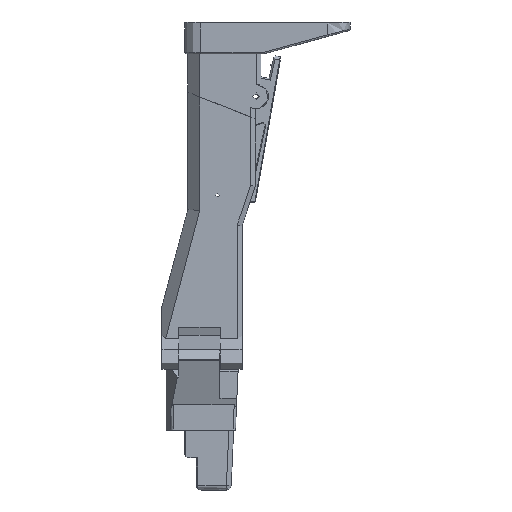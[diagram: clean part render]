
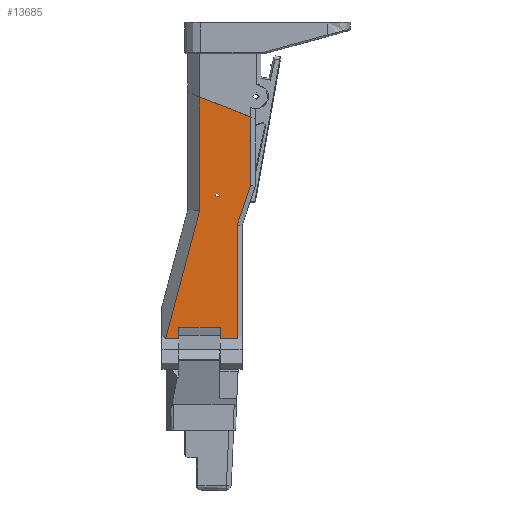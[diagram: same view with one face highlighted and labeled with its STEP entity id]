
A CAD part, left-side view. The second image highlights one B-rep face of the part: STEP entity #13685.
In plain terms, the highlighted planar face has unit normal (-1, 0, 0).
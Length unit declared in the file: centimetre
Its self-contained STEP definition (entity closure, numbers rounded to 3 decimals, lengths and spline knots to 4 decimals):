
#276=FACE_BOUND($,#2141,.T.);
#776=CIRCLE($,#14770,0.11);
#1345=FACE_OUTER_BOUND($,#2140,.T.);
#2140=EDGE_LOOP($,(#10818,#10819,#10820,#10821,#10822,#10823,#10824,#10825,
#10826,#10827,#10828));
#2141=EDGE_LOOP($,(#10829));
#3282=LINE($,#21640,#4736);
#3329=LINE($,#21742,#4783);
#3330=LINE($,#21744,#4784);
#3331=LINE($,#21746,#4785);
#3332=LINE($,#21748,#4786);
#3333=LINE($,#21750,#4787);
#3334=LINE($,#21752,#4788);
#3335=LINE($,#21754,#4789);
#3336=LINE($,#21756,#4790);
#3337=LINE($,#21758,#4791);
#3338=LINE($,#21759,#4792);
#4736=VECTOR($,#17386,3.427);
#4783=VECTOR($,#17457,7.1665);
#4784=VECTOR($,#17458,8.3408);
#4785=VECTOR($,#17459,0.8238);
#4786=VECTOR($,#17460,0.7375);
#4787=VECTOR($,#17461,2.61);
#4788=VECTOR($,#17462,0.7375);
#4789=VECTOR($,#17463,1.075);
#4790=VECTOR($,#17464,7.1624);
#4791=VECTOR($,#17465,2.631);
#4792=VECTOR($,#17466,4.2997);
#6103=VERTEX_POINT($,#21637);
#6104=VERTEX_POINT($,#21639);
#6147=VERTEX_POINT($,#21741);
#6148=VERTEX_POINT($,#21743);
#6149=VERTEX_POINT($,#21745);
#6150=VERTEX_POINT($,#21747);
#6151=VERTEX_POINT($,#21749);
#6152=VERTEX_POINT($,#21751);
#6153=VERTEX_POINT($,#21753);
#6154=VERTEX_POINT($,#21755);
#6155=VERTEX_POINT($,#21757);
#6156=VERTEX_POINT($,#21760);
#7762=EDGE_CURVE($,#6103,#6104,#3282,.T.);
#7813=EDGE_CURVE($,#6103,#6147,#3329,.T.);
#7814=EDGE_CURVE($,#6147,#6148,#3330,.T.);
#7815=EDGE_CURVE($,#6148,#6149,#3331,.T.);
#7816=EDGE_CURVE($,#6150,#6149,#3332,.T.);
#7817=EDGE_CURVE($,#6151,#6150,#3333,.T.);
#7818=EDGE_CURVE($,#6152,#6151,#3334,.T.);
#7819=EDGE_CURVE($,#6152,#6153,#3335,.T.);
#7820=EDGE_CURVE($,#6153,#6154,#3336,.T.);
#7821=EDGE_CURVE($,#6154,#6155,#3337,.T.);
#7822=EDGE_CURVE($,#6155,#6104,#3338,.T.);
#7823=EDGE_CURVE($,#6156,#6156,#776,.T.);
#10818=ORIENTED_EDGE($,*,*,#7762,.F.);
#10819=ORIENTED_EDGE($,*,*,#7813,.T.);
#10820=ORIENTED_EDGE($,*,*,#7814,.T.);
#10821=ORIENTED_EDGE($,*,*,#7815,.T.);
#10822=ORIENTED_EDGE($,*,*,#7816,.F.);
#10823=ORIENTED_EDGE($,*,*,#7817,.F.);
#10824=ORIENTED_EDGE($,*,*,#7818,.F.);
#10825=ORIENTED_EDGE($,*,*,#7819,.T.);
#10826=ORIENTED_EDGE($,*,*,#7820,.T.);
#10827=ORIENTED_EDGE($,*,*,#7821,.T.);
#10828=ORIENTED_EDGE($,*,*,#7822,.T.);
#10829=ORIENTED_EDGE($,*,*,#7823,.F.);
#13016=PLANE($,#14769);
#13685=ADVANCED_FACE($,(#1345,#276),#13016,.F.);
#14769=AXIS2_PLACEMENT_3D($,#21740,#17455,#17456);
#14770=AXIS2_PLACEMENT_3D($,#21761,#17467,#17468);
#17386=DIRECTION($,(0.,-0.929,-0.369));
#17455=DIRECTION('center_axis',(1.,0.,0.));
#17456=DIRECTION('ref_axis',(0.,0.,
-1.));
#17457=DIRECTION($,(0.,0.,-1.));
#17458=DIRECTION($,(0.,0.257,-0.966));
#17459=DIRECTION($,(0.,-1.,0.));
#17460=DIRECTION($,(0.,0.,-1.));
#17461=DIRECTION($,(0.,1.,0.));
#17462=DIRECTION($,(0.,0.,1.));
#17463=DIRECTION($,(0.,-1.,0.));
#17464=DIRECTION($,(0.,0.,1.));
#17465=DIRECTION($,(0.,-0.312,0.95));
#17466=DIRECTION($,(0.,0.,1.));
#17467=DIRECTION('center_axis',(-1.,0.,0.));
#17468=DIRECTION('ref_axis',(0.,0.,
1.));
#21637=CARTESIAN_POINT('',(-1.529,-2.1081,46.7504));
#21639=CARTESIAN_POINT('',(-1.529,-5.2931,45.4854));
#21640=CARTESIAN_POINT($,(-1.529,-6.9022,44.8463));
#21740=CARTESIAN_POINT('Origin',(-1.529,-4.7731,29.6912));
#21741=CARTESIAN_POINT('',(-1.529,-2.1081,39.5838));
#21742=CARTESIAN_POINT($,(-1.529,-2.1081,38.9412));
#21743=CARTESIAN_POINT('',(-1.529,0.0357,31.5233));
#21744=CARTESIAN_POINT($,(-1.529,-0.955,35.2482));
#21745=CARTESIAN_POINT('',(-1.529,-0.7881,31.5233));
#21746=CARTESIAN_POINT($,(-1.529,-2.0981,31.5233));
#21747=CARTESIAN_POINT('',(-1.529,-0.7881,32.2608));
#21748=CARTESIAN_POINT($,(-1.529,-0.7881,27.9643));
#21749=CARTESIAN_POINT('',(-1.529,-3.3981,32.2608));
#21750=CARTESIAN_POINT($,(-1.529,-2.7806,32.2608));
#21751=CARTESIAN_POINT('',(-1.529,-3.3981,31.5233));
#21752=CARTESIAN_POINT($,(-1.529,-3.3981,27.9836));
#21753=CARTESIAN_POINT('',(-1.529,-4.4731,31.5233));
#21754=CARTESIAN_POINT($,(-1.529,-4.7731,31.5233));
#21755=CARTESIAN_POINT('',(-1.529,-4.4731,38.6856));
#21756=CARTESIAN_POINT($,(-1.529,-4.4731,29.6912));
#21757=CARTESIAN_POINT('',(-1.529,-5.2931,41.1856));
#21758=CARTESIAN_POINT($,(-1.529,-3.1633,34.6925));
#21759=CARTESIAN_POINT($,(-1.529,-5.2931,46.3112));
#21760=CARTESIAN_POINT('',(-1.529,-3.2181,40.4562));
#21761=CARTESIAN_POINT('Origin',(-1.529,-3.2181,40.5662));
